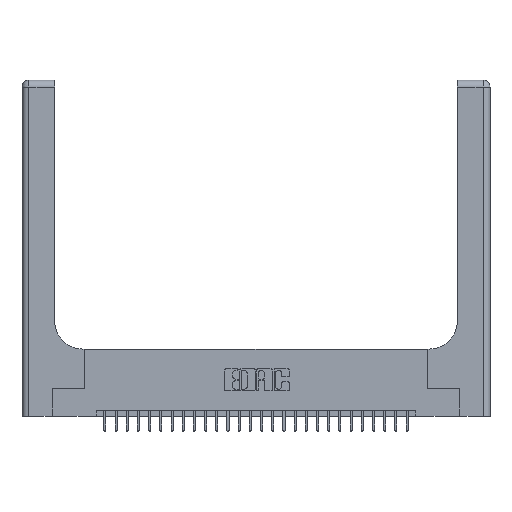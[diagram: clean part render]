
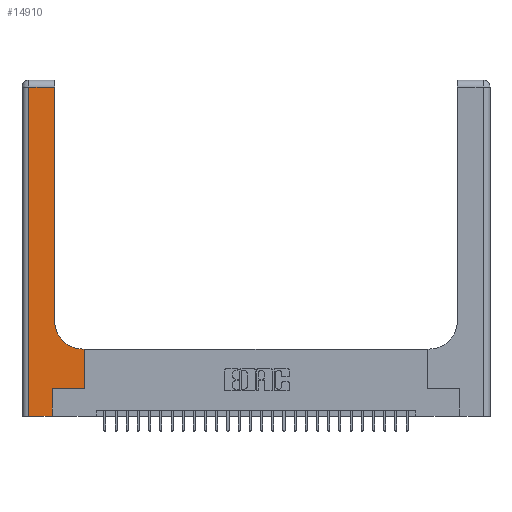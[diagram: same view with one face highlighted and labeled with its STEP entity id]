
A CAD part, top view. The second image highlights one B-rep face of the part: STEP entity #14910.
In plain terms, the highlighted planar face has unit normal (0, 0, 1).
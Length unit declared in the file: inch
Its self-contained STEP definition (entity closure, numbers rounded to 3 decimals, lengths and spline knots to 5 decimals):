
#44 = ORIENTED_EDGE ( 'NONE', *, *, #7297, .T. ) ;
#92 = EDGE_LOOP ( 'NONE', ( #4026, #16943, #19060, #14066, #25464, #12649, #16243, #5889, #44 ) ) ;
#476 = CARTESIAN_POINT ( 'NONE',  ( 0.2915, 0.85, 0.37 ) ) ;
#691 = VECTOR ( 'NONE', #949, 39.37008 ) ;
#932 = CARTESIAN_POINT ( 'NONE',  ( 0.5585, 0.6, 0.37 ) ) ;
#949 = DIRECTION ( 'NONE',  ( 1., 0., 0. ) ) ;
#1384 = LINE ( 'NONE', #3597, #691 ) ;
#1634 = CARTESIAN_POINT ( 'NONE',  ( 0.269, 0.25, 0.37 ) ) ;
#1950 = EDGE_CURVE ( 'NONE', #21971, #10962, #16235, .T. ) ;
#2434 = DIRECTION ( 'NONE',  ( -1., 0., 0. ) ) ;
#2596 = CARTESIAN_POINT ( 'NONE',  ( 0.2915, 3., 0.37 ) ) ;
#3354 = LINE ( 'NONE', #25729, #12072 ) ;
#3597 = CARTESIAN_POINT ( 'NONE',  ( 0.269, 0.25, 0.37 ) ) ;
#4026 = ORIENTED_EDGE ( 'NONE', *, *, #26023, .T. ) ;
#4488 = PLANE ( 'NONE',  #18846 ) ;
#4642 = DIRECTION ( 'NONE',  ( -1., 0., 0. ) ) ;
#4974 = DIRECTION ( 'NONE',  ( 0., 1., 0. ) ) ;
#5190 = EDGE_CURVE ( 'NONE', #10962, #24733, #24997, .T. ) ;
#5889 = ORIENTED_EDGE ( 'NONE', *, *, #5190, .T. ) ;
#6560 = DIRECTION ( 'NONE',  ( 0., 0., -1. ) ) ;
#7122 = CIRCLE ( 'NONE', #28806, 0.25 ) ;
#7129 = CARTESIAN_POINT ( 'NONE',  ( 0., 0., 0.37 ) ) ;
#7175 = VERTEX_POINT ( 'NONE', #23117 ) ;
#7192 = LINE ( 'NONE', #2596, #12511 ) ;
#7267 = DIRECTION ( 'NONE',  ( 0., -1., 0. ) ) ;
#7297 = EDGE_CURVE ( 'NONE', #24733, #16216, #7122, .T. ) ;
#7995 = VERTEX_POINT ( 'NONE', #22887 ) ;
#8198 = CARTESIAN_POINT ( 'NONE',  ( 0.2915, 2.94, 0.37 ) ) ;
#8247 = VECTOR ( 'NONE', #14119, 39.37008 ) ;
#8606 = CARTESIAN_POINT ( 'NONE',  ( 0.5585, 0.25, 0.37 ) ) ;
#8766 = DIRECTION ( 'NONE',  ( 0., 0., -1. ) ) ;
#9178 = LINE ( 'NONE', #7129, #12885 ) ;
#10649 = VERTEX_POINT ( 'NONE', #8198 ) ;
#10962 = VERTEX_POINT ( 'NONE', #932 ) ;
#11942 = CARTESIAN_POINT ( 'NONE',  ( 0.06, 2.94, 0.37 ) ) ;
#12072 = VECTOR ( 'NONE', #18958, 39.37008 ) ;
#12511 = VECTOR ( 'NONE', #4974, 39.37008 ) ;
#12513 = LINE ( 'NONE', #21485, #8247 ) ;
#12649 = ORIENTED_EDGE ( 'NONE', *, *, #21795, .T. ) ;
#12795 = VECTOR ( 'NONE', #2434, 39.37008 ) ;
#12885 = VECTOR ( 'NONE', #18147, 39.37008 ) ;
#13262 = CARTESIAN_POINT ( 'NONE',  ( 0.5415, 0.6, 0.37 ) ) ;
#13332 = FACE_OUTER_BOUND ( 'NONE', #92, .T. ) ;
#13472 = CARTESIAN_POINT ( 'NONE',  ( 0., 3., 0.37 ) ) ;
#14066 = ORIENTED_EDGE ( 'NONE', *, *, #23862, .T. ) ;
#14119 = DIRECTION ( 'NONE',  ( 0., 1., 0. ) ) ;
#14910 = ADVANCED_FACE ( 'NONE', ( #13332 ), #4488, .F. ) ;
#15677 = CARTESIAN_POINT ( 'NONE',  ( 0.2915, 0.6, 0.37 ) ) ;
#16216 = VERTEX_POINT ( 'NONE', #476 ) ;
#16235 = LINE ( 'NONE', #25110, #21602 ) ;
#16243 = ORIENTED_EDGE ( 'NONE', *, *, #1950, .T. ) ;
#16943 = ORIENTED_EDGE ( 'NONE', *, *, #26941, .T. ) ;
#17731 = DIRECTION ( 'NONE',  ( 1., 0., 0. ) ) ;
#18055 = VECTOR ( 'NONE', #7267, 39.37008 ) ;
#18147 = DIRECTION ( 'NONE',  ( 1., 0., 0. ) ) ;
#18480 = VERTEX_POINT ( 'NONE', #1634 ) ;
#18846 = AXIS2_PLACEMENT_3D ( 'NONE', #13472, #8766, #4642 ) ;
#18958 = DIRECTION ( 'NONE',  ( -1., 0., 0. ) ) ;
#19060 = ORIENTED_EDGE ( 'NONE', *, *, #24448, .T. ) ;
#20416 = CARTESIAN_POINT ( 'NONE',  ( 0.5415, 0.85, 0.37 ) ) ;
#21485 = CARTESIAN_POINT ( 'NONE',  ( 0.269, 0., 0.37 ) ) ;
#21602 = VECTOR ( 'NONE', #22752, 39.37008 ) ;
#21795 = EDGE_CURVE ( 'NONE', #18480, #21971, #1384, .T. ) ;
#21971 = VERTEX_POINT ( 'NONE', #8606 ) ;
#22740 = LINE ( 'NONE', #25101, #18055 ) ;
#22752 = DIRECTION ( 'NONE',  ( 0., 1., 0. ) ) ;
#22887 = CARTESIAN_POINT ( 'NONE',  ( 0.269, 0., 0.37 ) ) ;
#23117 = CARTESIAN_POINT ( 'NONE',  ( 0.06, 0., 0.37 ) ) ;
#23862 = EDGE_CURVE ( 'NONE', #7175, #7995, #9178, .T. ) ;
#24448 = EDGE_CURVE ( 'NONE', #25710, #7175, #22740, .T. ) ;
#24733 = VERTEX_POINT ( 'NONE', #13262 ) ;
#24997 = LINE ( 'NONE', #15677, #12795 ) ;
#25101 = CARTESIAN_POINT ( 'NONE',  ( 0.06, 3., 0.37 ) ) ;
#25110 = CARTESIAN_POINT ( 'NONE',  ( 0.5585, 0.25, 0.37 ) ) ;
#25464 = ORIENTED_EDGE ( 'NONE', *, *, #25836, .T. ) ;
#25710 = VERTEX_POINT ( 'NONE', #11942 ) ;
#25729 = CARTESIAN_POINT ( 'NONE',  ( 0., 2.94, 0.37 ) ) ;
#25836 = EDGE_CURVE ( 'NONE', #7995, #18480, #12513, .T. ) ;
#26023 = EDGE_CURVE ( 'NONE', #16216, #10649, #7192, .T. ) ;
#26941 = EDGE_CURVE ( 'NONE', #10649, #25710, #3354, .T. ) ;
#28806 = AXIS2_PLACEMENT_3D ( 'NONE', #20416, #6560, #17731 ) ;
